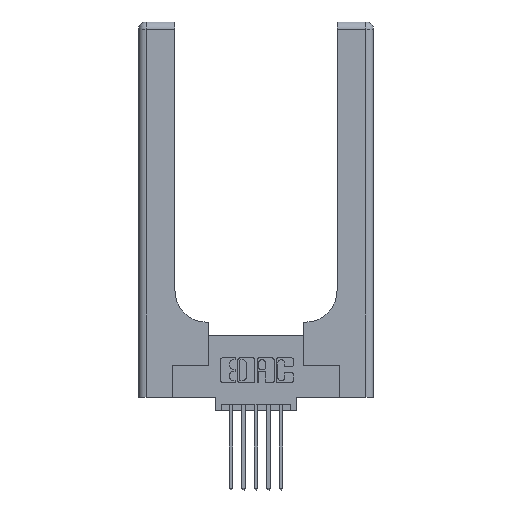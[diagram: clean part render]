
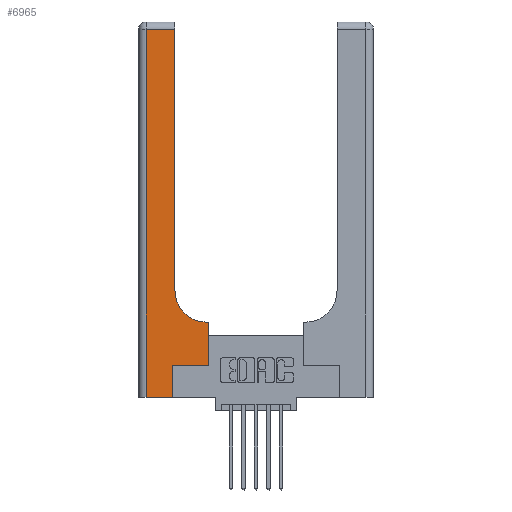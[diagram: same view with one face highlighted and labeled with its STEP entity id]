
A CAD part, top view. The second image highlights one B-rep face of the part: STEP entity #6965.
In plain terms, the highlighted planar face has unit normal (0, 0, 1).
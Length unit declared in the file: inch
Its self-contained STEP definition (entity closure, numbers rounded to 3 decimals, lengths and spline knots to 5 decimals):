
#40 = ORIENTED_EDGE ( 'NONE', *, *, #6288, .T. ) ;
#178 = VECTOR ( 'NONE', #12463, 39.37008 ) ;
#189 = VECTOR ( 'NONE', #4666, 39.37008 ) ;
#944 = CARTESIAN_POINT ( 'NONE',  ( 0.5585, 0.6, 0.37 ) ) ;
#1054 = DIRECTION ( 'NONE',  ( 0., 1., 0. ) ) ;
#1151 = VERTEX_POINT ( 'NONE', #2988 ) ;
#1321 = DIRECTION ( 'NONE',  ( 0., 1., 0. ) ) ;
#1350 = AXIS2_PLACEMENT_3D ( 'NONE', #5442, #5486, #5483 ) ;
#1485 = VECTOR ( 'NONE', #2298, 39.37008 ) ;
#1576 = LINE ( 'NONE', #5620, #10046 ) ;
#1627 = CARTESIAN_POINT ( 'NONE',  ( 0.2915, 0.85, 0.37 ) ) ;
#2298 = DIRECTION ( 'NONE',  ( 0., -1., 0. ) ) ;
#2456 = VECTOR ( 'NONE', #6709, 39.37008 ) ;
#2988 = CARTESIAN_POINT ( 'NONE',  ( 0.06, 2.94, 0.37 ) ) ;
#3083 = VECTOR ( 'NONE', #1321, 39.37008 ) ;
#3495 = VERTEX_POINT ( 'NONE', #3946 ) ;
#3607 = DIRECTION ( 'NONE',  ( -1., 0., 0. ) ) ;
#3815 = LINE ( 'NONE', #4777, #3083 ) ;
#3946 = CARTESIAN_POINT ( 'NONE',  ( 0.269, 0.25, 0.37 ) ) ;
#3972 = ORIENTED_EDGE ( 'NONE', *, *, #8742, .T. ) ;
#4092 = EDGE_LOOP ( 'NONE', ( #8441, #11296, #8767, #11981, #3972, #13002, #40, #9261, #6745 ) ) ;
#4541 = LINE ( 'NONE', #11078, #1485 ) ;
#4666 = DIRECTION ( 'NONE',  ( -1., 0., 0. ) ) ;
#4756 = CARTESIAN_POINT ( 'NONE',  ( 0., 2.94, 0.37 ) ) ;
#4777 = CARTESIAN_POINT ( 'NONE',  ( 0.269, 0., 0.37 ) ) ;
#5026 = EDGE_CURVE ( 'NONE', #10157, #7832, #10949, .T. ) ;
#5442 = CARTESIAN_POINT ( 'NONE',  ( 0.5415, 0.85, 0.37 ) ) ;
#5483 = DIRECTION ( 'NONE',  ( 1., 0., 0. ) ) ;
#5486 = DIRECTION ( 'NONE',  ( 0., 0., -1. ) ) ;
#5503 = LINE ( 'NONE', #9895, #2456 ) ;
#5620 = CARTESIAN_POINT ( 'NONE',  ( 0.2915, 3., 0.37 ) ) ;
#5642 = DIRECTION ( 'NONE',  ( -1., 0., 0. ) ) ;
#5673 = CARTESIAN_POINT ( 'NONE',  ( 0.2915, 2.94, 0.37 ) ) ;
#5732 = DIRECTION ( 'NONE',  ( 0., 0., -1. ) ) ;
#6157 = VECTOR ( 'NONE', #12705, 39.37008 ) ;
#6187 = LINE ( 'NONE', #7932, #189 ) ;
#6246 = PLANE ( 'NONE',  #9606 ) ;
#6288 = EDGE_CURVE ( 'NONE', #8991, #10492, #9054, .T. ) ;
#6709 = DIRECTION ( 'NONE',  ( 1., 0., 0. ) ) ;
#6745 = ORIENTED_EDGE ( 'NONE', *, *, #5026, .T. ) ;
#6965 = ADVANCED_FACE ( 'NONE', ( #12962 ), #6246, .F. ) ;
#7487 = EDGE_CURVE ( 'NONE', #7832, #11686, #1576, .T. ) ;
#7832 = VERTEX_POINT ( 'NONE', #1627 ) ;
#7932 = CARTESIAN_POINT ( 'NONE',  ( 0.2915, 0.6, 0.37 ) ) ;
#8188 = CARTESIAN_POINT ( 'NONE',  ( 0.269, 0., 0.37 ) ) ;
#8231 = CARTESIAN_POINT ( 'NONE',  ( 0., 3., 0.37 ) ) ;
#8373 = CARTESIAN_POINT ( 'NONE',  ( 0., 0., 0.37 ) ) ;
#8441 = ORIENTED_EDGE ( 'NONE', *, *, #7487, .T. ) ;
#8500 = VERTEX_POINT ( 'NONE', #9731 ) ;
#8668 = EDGE_CURVE ( 'NONE', #1151, #8500, #4541, .T. ) ;
#8742 = EDGE_CURVE ( 'NONE', #12520, #3495, #3815, .T. ) ;
#8767 = ORIENTED_EDGE ( 'NONE', *, *, #8668, .T. ) ;
#8991 = VERTEX_POINT ( 'NONE', #9440 ) ;
#9054 = LINE ( 'NONE', #12561, #178 ) ;
#9261 = ORIENTED_EDGE ( 'NONE', *, *, #11708, .T. ) ;
#9353 = EDGE_CURVE ( 'NONE', #11686, #1151, #10109, .T. ) ;
#9357 = LINE ( 'NONE', #8373, #6157 ) ;
#9440 = CARTESIAN_POINT ( 'NONE',  ( 0.5585, 0.25, 0.37 ) ) ;
#9606 = AXIS2_PLACEMENT_3D ( 'NONE', #8231, #5732, #5642 ) ;
#9731 = CARTESIAN_POINT ( 'NONE',  ( 0.06, 0., 0.37 ) ) ;
#9895 = CARTESIAN_POINT ( 'NONE',  ( 0.269, 0.25, 0.37 ) ) ;
#10046 = VECTOR ( 'NONE', #1054, 39.37008 ) ;
#10109 = LINE ( 'NONE', #4756, #13347 ) ;
#10157 = VERTEX_POINT ( 'NONE', #13469 ) ;
#10492 = VERTEX_POINT ( 'NONE', #944 ) ;
#10949 = CIRCLE ( 'NONE', #1350, 0.25 ) ;
#11078 = CARTESIAN_POINT ( 'NONE',  ( 0.06, 3., 0.37 ) ) ;
#11296 = ORIENTED_EDGE ( 'NONE', *, *, #9353, .T. ) ;
#11686 = VERTEX_POINT ( 'NONE', #5673 ) ;
#11708 = EDGE_CURVE ( 'NONE', #10492, #10157, #6187, .T. ) ;
#11981 = ORIENTED_EDGE ( 'NONE', *, *, #12626, .T. ) ;
#12258 = EDGE_CURVE ( 'NONE', #3495, #8991, #5503, .T. ) ;
#12463 = DIRECTION ( 'NONE',  ( 0., 1., 0. ) ) ;
#12520 = VERTEX_POINT ( 'NONE', #8188 ) ;
#12561 = CARTESIAN_POINT ( 'NONE',  ( 0.5585, 0.25, 0.37 ) ) ;
#12626 = EDGE_CURVE ( 'NONE', #8500, #12520, #9357, .T. ) ;
#12705 = DIRECTION ( 'NONE',  ( 1., 0., 0. ) ) ;
#12962 = FACE_OUTER_BOUND ( 'NONE', #4092, .T. ) ;
#13002 = ORIENTED_EDGE ( 'NONE', *, *, #12258, .T. ) ;
#13347 = VECTOR ( 'NONE', #3607, 39.37008 ) ;
#13469 = CARTESIAN_POINT ( 'NONE',  ( 0.5415, 0.6, 0.37 ) ) ;
